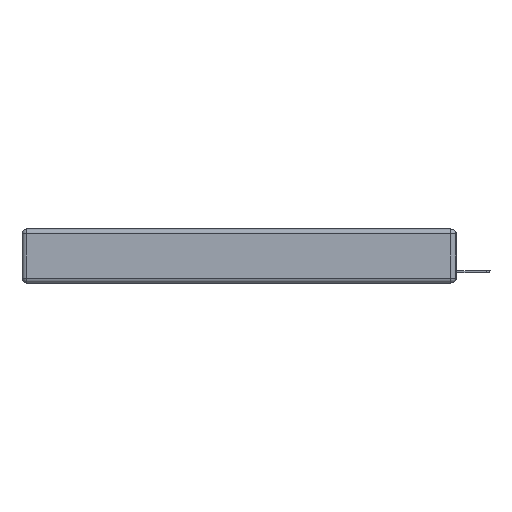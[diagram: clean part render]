
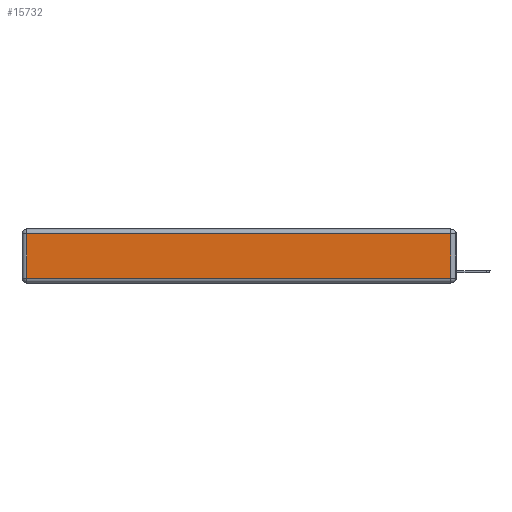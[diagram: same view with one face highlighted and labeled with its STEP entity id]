
A CAD part, left-side view. The second image highlights one B-rep face of the part: STEP entity #15732.
In plain terms, the highlighted planar face has unit normal (-1, 0, 0).
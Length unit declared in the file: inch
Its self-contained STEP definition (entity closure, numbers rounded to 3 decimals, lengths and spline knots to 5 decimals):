
#1174 = CARTESIAN_POINT ( 'NONE',  ( 0., 2.72, -0.313 ) ) ;
#1283 = EDGE_CURVE ( 'NONE', #10316, #6365, #12966, .T. ) ;
#1805 = DIRECTION ( 'NONE',  ( -1., 0., 0. ) ) ;
#1824 = ORIENTED_EDGE ( 'NONE', *, *, #10506, .T. ) ;
#2102 = VECTOR ( 'NONE', #8615, 39.37008 ) ;
#3013 = ORIENTED_EDGE ( 'NONE', *, *, #13919, .T. ) ;
#3249 = CARTESIAN_POINT ( 'NONE',  ( 0., 0., -0.343 ) ) ;
#3914 = LINE ( 'NONE', #7201, #2102 ) ;
#4706 = CARTESIAN_POINT ( 'NONE',  ( 0., 0., -0.313 ) ) ;
#6365 = VERTEX_POINT ( 'NONE', #11183 ) ;
#6511 = ORIENTED_EDGE ( 'NONE', *, *, #16960, .T. ) ;
#6945 = VERTEX_POINT ( 'NONE', #12646 ) ;
#7201 = CARTESIAN_POINT ( 'NONE',  ( 0., 2.75, -0.03 ) ) ;
#7369 = VECTOR ( 'NONE', #10642, 39.37008 ) ;
#7566 = PLANE ( 'NONE',  #15272 ) ;
#7625 = DIRECTION ( 'NONE',  ( 0., 0., 1. ) ) ;
#7721 = VECTOR ( 'NONE', #11795, 39.37008 ) ;
#7796 = CARTESIAN_POINT ( 'NONE',  ( 0., 0.03, -0.343 ) ) ;
#8615 = DIRECTION ( 'NONE',  ( 0., 1., 0. ) ) ;
#9053 = LINE ( 'NONE', #17485, #7721 ) ;
#9403 = FACE_OUTER_BOUND ( 'NONE', #14421, .T. ) ;
#9692 = ORIENTED_EDGE ( 'NONE', *, *, #1283, .T. ) ;
#10316 = VERTEX_POINT ( 'NONE', #1174 ) ;
#10506 = EDGE_CURVE ( 'NONE', #6945, #11854, #3914, .T. ) ;
#10642 = DIRECTION ( 'NONE',  ( 0., 0., 1. ) ) ;
#11183 = CARTESIAN_POINT ( 'NONE',  ( 0., 0.03, -0.313 ) ) ;
#11422 = VECTOR ( 'NONE', #14783, 39.37008 ) ;
#11795 = DIRECTION ( 'NONE',  ( 0., 0., -1. ) ) ;
#11854 = VERTEX_POINT ( 'NONE', #12969 ) ;
#12646 = CARTESIAN_POINT ( 'NONE',  ( 0., 0.03, -0.03 ) ) ;
#12966 = LINE ( 'NONE', #4706, #11422 ) ;
#12969 = CARTESIAN_POINT ( 'NONE',  ( 0., 2.72, -0.03 ) ) ;
#13919 = EDGE_CURVE ( 'NONE', #11854, #10316, #9053, .T. ) ;
#14255 = LINE ( 'NONE', #7796, #7369 ) ;
#14421 = EDGE_LOOP ( 'NONE', ( #9692, #6511, #1824, #3013 ) ) ;
#14783 = DIRECTION ( 'NONE',  ( 0., -1., 0. ) ) ;
#15272 = AXIS2_PLACEMENT_3D ( 'NONE', #3249, #1805, #7625 ) ;
#15732 = ADVANCED_FACE ( 'NONE', ( #9403 ), #7566, .T. ) ;
#16960 = EDGE_CURVE ( 'NONE', #6365, #6945, #14255, .T. ) ;
#17485 = CARTESIAN_POINT ( 'NONE',  ( 0., 2.72, -0.343 ) ) ;
